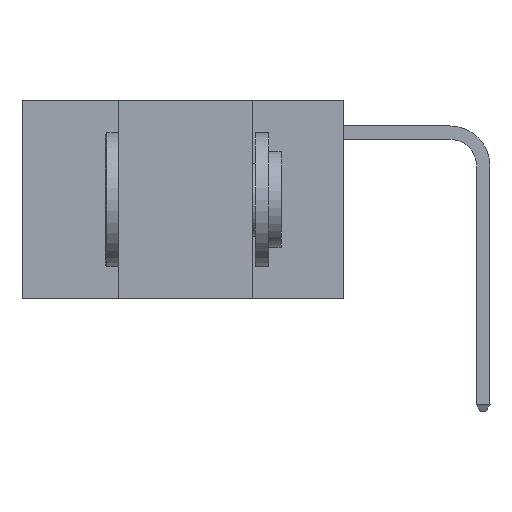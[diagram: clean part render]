
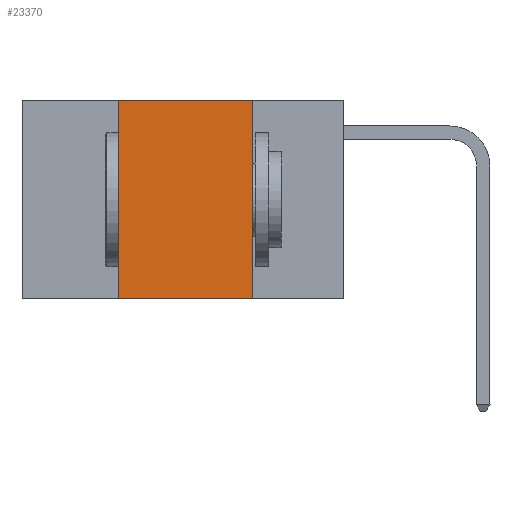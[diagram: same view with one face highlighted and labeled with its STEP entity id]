
A CAD part, left-side view. The second image highlights one B-rep face of the part: STEP entity #23370.
In plain terms, the highlighted planar face has unit normal (-1, 0, 0).
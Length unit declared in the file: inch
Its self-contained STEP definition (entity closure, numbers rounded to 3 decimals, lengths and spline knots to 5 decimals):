
#20 = CARTESIAN_POINT ( 'NONE',  ( 0., 0.17, -0.37 ) ) ;
#495 = LINE ( 'NONE', #11909, #867 ) ;
#867 = VECTOR ( 'NONE', #6166, 39.37008 ) ;
#1024 = AXIS2_PLACEMENT_3D ( 'NONE', #1162, #20245, #18502 ) ;
#1162 = CARTESIAN_POINT ( 'NONE',  ( 0., 0.6, 0. ) ) ;
#1496 = VERTEX_POINT ( 'NONE', #10763 ) ;
#1738 = LINE ( 'NONE', #5346, #4021 ) ;
#2114 = ORIENTED_EDGE ( 'NONE', *, *, #3976, .F. ) ;
#2455 = CARTESIAN_POINT ( 'NONE',  ( 0., 0.17, 0. ) ) ;
#3616 = EDGE_CURVE ( 'NONE', #1496, #23831, #8491, .T. ) ;
#3769 = LINE ( 'NONE', #22933, #5150 ) ;
#3976 = EDGE_CURVE ( 'NONE', #21406, #1496, #3769, .T. ) ;
#4021 = VECTOR ( 'NONE', #15021, 39.37008 ) ;
#5150 = VECTOR ( 'NONE', #9688, 39.37008 ) ;
#5346 = CARTESIAN_POINT ( 'NONE',  ( 0., 0.42, 0. ) ) ;
#5963 = EDGE_CURVE ( 'NONE', #13374, #21406, #1738, .T. ) ;
#6166 = DIRECTION ( 'NONE',  ( 0., -1., 0. ) ) ;
#6778 = EDGE_CURVE ( 'NONE', #13374, #23831, #495, .T. ) ;
#8491 = LINE ( 'NONE', #2455, #24119 ) ;
#8829 = FACE_OUTER_BOUND ( 'NONE', #19791, .T. ) ;
#9043 = CARTESIAN_POINT ( 'NONE',  ( 0., 0.42, -0.37 ) ) ;
#9688 = DIRECTION ( 'NONE',  ( 0., -1., 0. ) ) ;
#10255 = ORIENTED_EDGE ( 'NONE', *, *, #6778, .T. ) ;
#10763 = CARTESIAN_POINT ( 'NONE',  ( 0., 0.17, 0. ) ) ;
#11486 = ORIENTED_EDGE ( 'NONE', *, *, #5963, .F. ) ;
#11909 = CARTESIAN_POINT ( 'NONE',  ( 0., 0.6, -0.37 ) ) ;
#13374 = VERTEX_POINT ( 'NONE', #9043 ) ;
#15021 = DIRECTION ( 'NONE',  ( 0., 0., 1. ) ) ;
#16060 = DIRECTION ( 'NONE',  ( 0., 0., -1. ) ) ;
#16839 = ORIENTED_EDGE ( 'NONE', *, *, #3616, .F. ) ;
#18502 = DIRECTION ( 'NONE',  ( 0., 0., -1. ) ) ;
#19791 = EDGE_LOOP ( 'NONE', ( #16839, #2114, #11486, #10255 ) ) ;
#20245 = DIRECTION ( 'NONE',  ( 1., 0., 0. ) ) ;
#20484 = PLANE ( 'NONE',  #1024 ) ;
#21406 = VERTEX_POINT ( 'NONE', #21637 ) ;
#21637 = CARTESIAN_POINT ( 'NONE',  ( 0., 0.42, 0. ) ) ;
#22933 = CARTESIAN_POINT ( 'NONE',  ( 0., 0.6, 0. ) ) ;
#23370 = ADVANCED_FACE ( 'NONE', ( #8829 ), #20484, .F. ) ;
#23831 = VERTEX_POINT ( 'NONE', #20 ) ;
#24119 = VECTOR ( 'NONE', #16060, 39.37008 ) ;
